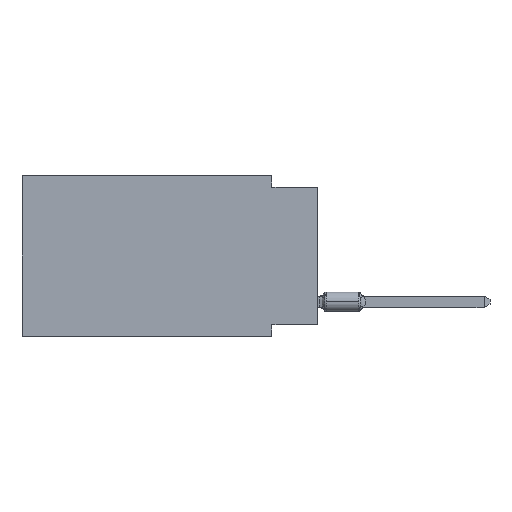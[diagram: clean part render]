
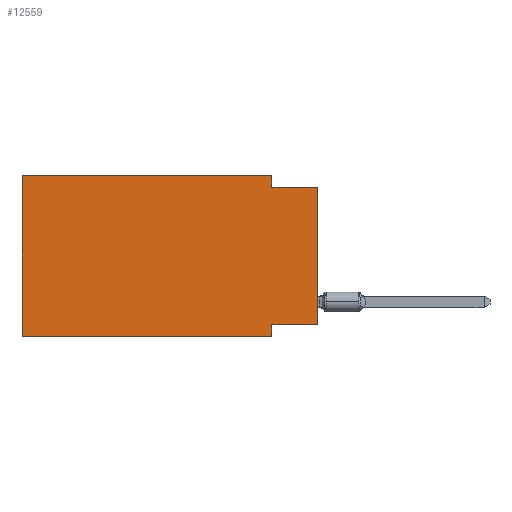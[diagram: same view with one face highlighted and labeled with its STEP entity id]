
A CAD part, left-side view. The second image highlights one B-rep face of the part: STEP entity #12559.
In plain terms, the highlighted planar face has unit normal (-1, 0, 0).
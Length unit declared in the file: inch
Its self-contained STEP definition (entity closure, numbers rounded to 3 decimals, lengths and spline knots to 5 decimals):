
#174 = CARTESIAN_POINT ( 'NONE',  ( 0., 0., -0.325 ) ) ;
#579 = VERTEX_POINT ( 'NONE', #11497 ) ;
#638 = EDGE_CURVE ( 'NONE', #6055, #8691, #6781, .T. ) ;
#661 = ORIENTED_EDGE ( 'NONE', *, *, #13567, .T. ) ;
#684 = AXIS2_PLACEMENT_3D ( 'NONE', #3218, #6481, #12475 ) ;
#1077 = LINE ( 'NONE', #6984, #1991 ) ;
#1100 = DIRECTION ( 'NONE',  ( 0., 1., 0. ) ) ;
#1231 = EDGE_CURVE ( 'NONE', #11417, #10949, #11921, .T. ) ;
#1330 = CARTESIAN_POINT ( 'NONE',  ( 0., 0., -0.325 ) ) ;
#1521 = ORIENTED_EDGE ( 'NONE', *, *, #9651, .F. ) ;
#1604 = VECTOR ( 'NONE', #10286, 39.37008 ) ;
#1991 = VECTOR ( 'NONE', #4637, 39.37008 ) ;
#2074 = CARTESIAN_POINT ( 'NONE',  ( 0., 0.1, -0.35 ) ) ;
#2442 = EDGE_CURVE ( 'NONE', #6468, #8691, #3889, .T. ) ;
#2670 = DIRECTION ( 'NONE',  ( 0., -1., 0. ) ) ;
#2673 = CARTESIAN_POINT ( 'NONE',  ( 0., 0.645, -0.35 ) ) ;
#3218 = CARTESIAN_POINT ( 'NONE',  ( 0., 0.645, 0. ) ) ;
#3561 = CARTESIAN_POINT ( 'NONE',  ( 0., 0.1, -0.025 ) ) ;
#3889 = LINE ( 'NONE', #14219, #10471 ) ;
#3967 = EDGE_CURVE ( 'NONE', #10949, #6055, #1077, .T. ) ;
#4100 = ORIENTED_EDGE ( 'NONE', *, *, #4900, .F. ) ;
#4637 = DIRECTION ( 'NONE',  ( 0., 0., -1. ) ) ;
#4900 = EDGE_CURVE ( 'NONE', #579, #11417, #13457, .T. ) ;
#5269 = CARTESIAN_POINT ( 'NONE',  ( 0., 0.645, 0. ) ) ;
#5320 = DIRECTION ( 'NONE',  ( 0., 0., 1. ) ) ;
#5843 = LINE ( 'NONE', #2673, #14753 ) ;
#6055 = VERTEX_POINT ( 'NONE', #3561 ) ;
#6297 = CARTESIAN_POINT ( 'NONE',  ( 0., 0.645, 0. ) ) ;
#6468 = VERTEX_POINT ( 'NONE', #1330 ) ;
#6481 = DIRECTION ( 'NONE',  ( 1., 0., 0. ) ) ;
#6781 = LINE ( 'NONE', #9138, #1604 ) ;
#6984 = CARTESIAN_POINT ( 'NONE',  ( 0., 0.1, 0. ) ) ;
#7235 = ORIENTED_EDGE ( 'NONE', *, *, #638, .F. ) ;
#7955 = ORIENTED_EDGE ( 'NONE', *, *, #2442, .T. ) ;
#8423 = ORIENTED_EDGE ( 'NONE', *, *, #3967, .F. ) ;
#8427 = DIRECTION ( 'NONE',  ( 0., -1., 0. ) ) ;
#8691 = VERTEX_POINT ( 'NONE', #12529 ) ;
#9025 = VECTOR ( 'NONE', #10201, 39.37008 ) ;
#9127 = PLANE ( 'NONE',  #684 ) ;
#9138 = CARTESIAN_POINT ( 'NONE',  ( 0., 0., -0.025 ) ) ;
#9292 = LINE ( 'NONE', #174, #9858 ) ;
#9651 = EDGE_CURVE ( 'NONE', #12743, #12011, #12471, .T. ) ;
#9858 = VECTOR ( 'NONE', #1100, 39.37008 ) ;
#10201 = DIRECTION ( 'NONE',  ( 0., 0., 1. ) ) ;
#10286 = DIRECTION ( 'NONE',  ( 0., -1., 0. ) ) ;
#10471 = VECTOR ( 'NONE', #5320, 39.37008 ) ;
#10590 = VECTOR ( 'NONE', #11332, 39.37008 ) ;
#10949 = VERTEX_POINT ( 'NONE', #14691 ) ;
#11072 = EDGE_CURVE ( 'NONE', #6468, #12743, #9292, .T. ) ;
#11332 = DIRECTION ( 'NONE',  ( 0., 0., -1. ) ) ;
#11417 = VERTEX_POINT ( 'NONE', #6297 ) ;
#11497 = CARTESIAN_POINT ( 'NONE',  ( 0., 0.645, -0.35 ) ) ;
#11505 = CARTESIAN_POINT ( 'NONE',  ( 0., 0.1, -0.35 ) ) ;
#11595 = VECTOR ( 'NONE', #2670, 39.37008 ) ;
#11886 = EDGE_LOOP ( 'NONE', ( #7955, #7235, #8423, #14328, #4100, #661, #1521, #14058 ) ) ;
#11921 = LINE ( 'NONE', #14346, #11595 ) ;
#12011 = VERTEX_POINT ( 'NONE', #11505 ) ;
#12471 = LINE ( 'NONE', #2074, #10590 ) ;
#12475 = DIRECTION ( 'NONE',  ( 0., 0., -1. ) ) ;
#12529 = CARTESIAN_POINT ( 'NONE',  ( 0., 0., -0.025 ) ) ;
#12559 = ADVANCED_FACE ( 'NONE', ( #13461 ), #9127, .F. ) ;
#12743 = VERTEX_POINT ( 'NONE', #14203 ) ;
#13457 = LINE ( 'NONE', #5269, #9025 ) ;
#13461 = FACE_OUTER_BOUND ( 'NONE', #11886, .T. ) ;
#13567 = EDGE_CURVE ( 'NONE', #579, #12011, #5843, .T. ) ;
#14058 = ORIENTED_EDGE ( 'NONE', *, *, #11072, .F. ) ;
#14203 = CARTESIAN_POINT ( 'NONE',  ( 0., 0.1, -0.325 ) ) ;
#14219 = CARTESIAN_POINT ( 'NONE',  ( 0., 0., 0. ) ) ;
#14328 = ORIENTED_EDGE ( 'NONE', *, *, #1231, .F. ) ;
#14346 = CARTESIAN_POINT ( 'NONE',  ( 0., 0.645, 0. ) ) ;
#14691 = CARTESIAN_POINT ( 'NONE',  ( 0., 0.1, 0. ) ) ;
#14753 = VECTOR ( 'NONE', #8427, 39.37008 ) ;
